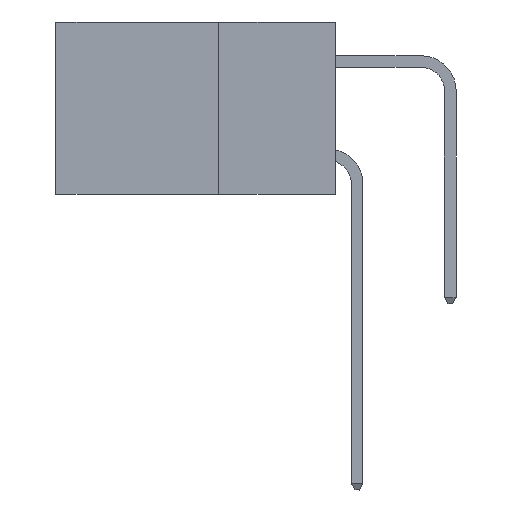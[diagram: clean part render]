
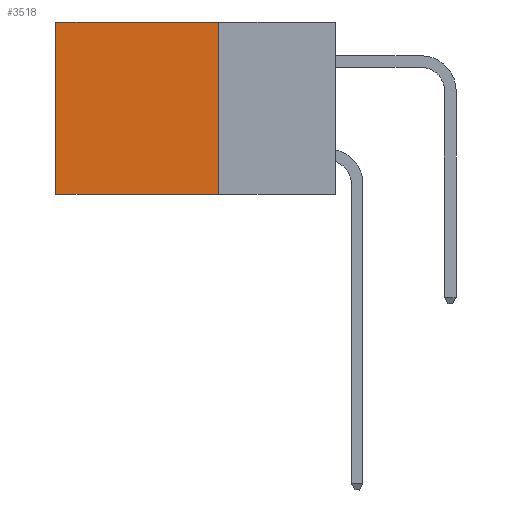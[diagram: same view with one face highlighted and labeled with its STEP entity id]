
A CAD part, left-side view. The second image highlights one B-rep face of the part: STEP entity #3518.
In plain terms, the highlighted planar face has unit normal (-1, 0, 0).
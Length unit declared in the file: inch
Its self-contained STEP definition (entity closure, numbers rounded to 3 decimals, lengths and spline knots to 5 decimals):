
#679 = DIRECTION ( 'NONE',  ( 0., 0., -1. ) ) ;
#1217 = EDGE_CURVE ( 'NONE', #9797, #14768, #6578, .T. ) ;
#2304 = LINE ( 'NONE', #2662, #3182 ) ;
#2662 = CARTESIAN_POINT ( 'NONE',  ( 0.2875, 0.25, -0.37 ) ) ;
#3182 = VECTOR ( 'NONE', #10259, 39.37008 ) ;
#3311 = VERTEX_POINT ( 'NONE', #21272 ) ;
#3518 = ADVANCED_FACE ( 'NONE', ( #12129 ), #21521, .F. ) ;
#3736 = ORIENTED_EDGE ( 'NONE', *, *, #1217, .T. ) ;
#4417 = CARTESIAN_POINT ( 'NONE',  ( 0.2875, 0.25, 0. ) ) ;
#4441 = AXIS2_PLACEMENT_3D ( 'NONE', #4417, #17777, #679 ) ;
#6578 = LINE ( 'NONE', #19931, #15053 ) ;
#6618 = LINE ( 'NONE', #6872, #16108 ) ;
#6832 = EDGE_CURVE ( 'NONE', #9797, #9941, #6618, .T. ) ;
#6872 = CARTESIAN_POINT ( 'NONE',  ( 0.2875, 0.25, 0. ) ) ;
#8214 = DIRECTION ( 'NONE',  ( 0., 1., 0. ) ) ;
#9729 = CARTESIAN_POINT ( 'NONE',  ( 0.2875, 0.25, -0.37 ) ) ;
#9797 = VERTEX_POINT ( 'NONE', #12596 ) ;
#9941 = VERTEX_POINT ( 'NONE', #9729 ) ;
#10259 = DIRECTION ( 'NONE',  ( 0., 1., 0. ) ) ;
#12129 = FACE_OUTER_BOUND ( 'NONE', #13164, .T. ) ;
#12596 = CARTESIAN_POINT ( 'NONE',  ( 0.2875, 0.25, 0. ) ) ;
#13164 = EDGE_LOOP ( 'NONE', ( #16296, #21394, #16726, #3736 ) ) ;
#14768 = VERTEX_POINT ( 'NONE', #16002 ) ;
#14853 = LINE ( 'NONE', #18850, #18753 ) ;
#15053 = VECTOR ( 'NONE', #8214, 39.37008 ) ;
#16002 = CARTESIAN_POINT ( 'NONE',  ( 0.2875, 0.6, 0. ) ) ;
#16108 = VECTOR ( 'NONE', #16613, 39.37008 ) ;
#16296 = ORIENTED_EDGE ( 'NONE', *, *, #18288, .T. ) ;
#16302 = EDGE_CURVE ( 'NONE', #9941, #3311, #2304, .T. ) ;
#16613 = DIRECTION ( 'NONE',  ( 0., 0., -1. ) ) ;
#16726 = ORIENTED_EDGE ( 'NONE', *, *, #6832, .F. ) ;
#17777 = DIRECTION ( 'NONE',  ( 1., 0., 0. ) ) ;
#18288 = EDGE_CURVE ( 'NONE', #14768, #3311, #14853, .T. ) ;
#18753 = VECTOR ( 'NONE', #22474, 39.37008 ) ;
#18850 = CARTESIAN_POINT ( 'NONE',  ( 0.2875, 0.6, 0. ) ) ;
#19931 = CARTESIAN_POINT ( 'NONE',  ( 0.2875, 0.25, 0. ) ) ;
#21272 = CARTESIAN_POINT ( 'NONE',  ( 0.2875, 0.6, -0.37 ) ) ;
#21394 = ORIENTED_EDGE ( 'NONE', *, *, #16302, .F. ) ;
#21521 = PLANE ( 'NONE',  #4441 ) ;
#22474 = DIRECTION ( 'NONE',  ( 0., 0., -1. ) ) ;
